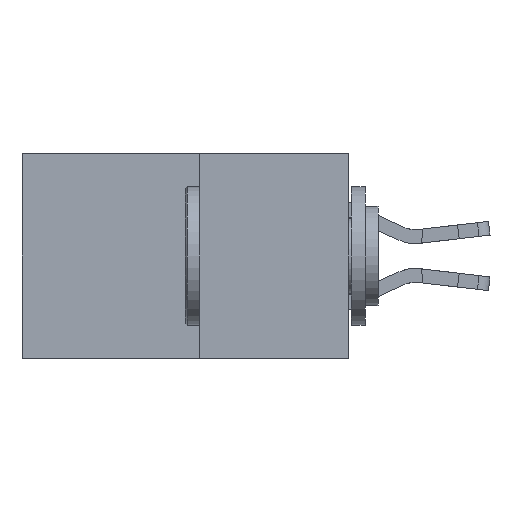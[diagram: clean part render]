
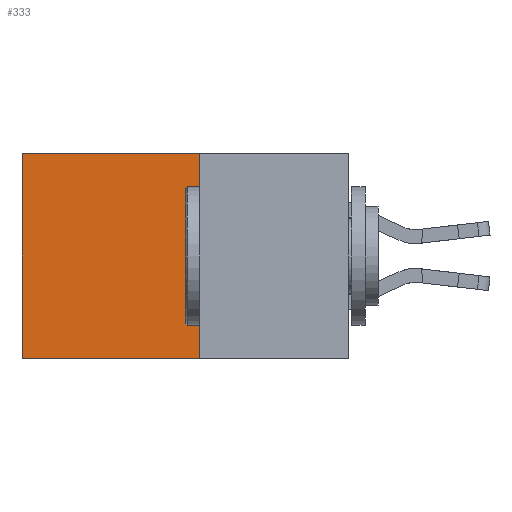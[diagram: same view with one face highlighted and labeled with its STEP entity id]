
A CAD part, left-side view. The second image highlights one B-rep face of the part: STEP entity #333.
In plain terms, the highlighted planar face has unit normal (-1, 0, 0).
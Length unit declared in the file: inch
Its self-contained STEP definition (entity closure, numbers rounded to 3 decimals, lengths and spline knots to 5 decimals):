
#333 = ADVANCED_FACE ( 'NONE', ( #1556 ), #15491, .F. ) ;
#645 = CARTESIAN_POINT ( 'NONE',  ( 0.277, 0.27, 0. ) ) ;
#831 = DIRECTION ( 'NONE',  ( 0., 0., -1. ) ) ;
#1556 = FACE_OUTER_BOUND ( 'NONE', #3323, .T. ) ;
#1983 = LINE ( 'NONE', #10233, #12766 ) ;
#2122 = EDGE_CURVE ( 'NONE', #16113, #11351, #10534, .T. ) ;
#2953 = CARTESIAN_POINT ( 'NONE',  ( 0.277, 0.59, -0.37 ) ) ;
#3068 = CARTESIAN_POINT ( 'NONE',  ( 0.277, 0.27, 0. ) ) ;
#3210 = VECTOR ( 'NONE', #16362, 39.37008 ) ;
#3323 = EDGE_LOOP ( 'NONE', ( #10973, #4220, #12655, #10870 ) ) ;
#3416 = CARTESIAN_POINT ( 'NONE',  ( 0.277, 0.27, -0.37 ) ) ;
#4220 = ORIENTED_EDGE ( 'NONE', *, *, #7150, .F. ) ;
#4374 = DIRECTION ( 'NONE',  ( 0., 1., 0. ) ) ;
#6694 = CARTESIAN_POINT ( 'NONE',  ( 0.277, 0.59, 0. ) ) ;
#7150 = EDGE_CURVE ( 'NONE', #10003, #11351, #1983, .T. ) ;
#7243 = DIRECTION ( 'NONE',  ( 1., 0., 0. ) ) ;
#7878 = VECTOR ( 'NONE', #11225, 39.37008 ) ;
#8454 = EDGE_CURVE ( 'NONE', #13635, #10003, #13472, .T. ) ;
#10003 = VERTEX_POINT ( 'NONE', #13019 ) ;
#10208 = DIRECTION ( 'NONE',  ( 0., 1., 0. ) ) ;
#10232 = EDGE_CURVE ( 'NONE', #13635, #16113, #10466, .T. ) ;
#10233 = CARTESIAN_POINT ( 'NONE',  ( 0.277, 0.27, -0.37 ) ) ;
#10466 = LINE ( 'NONE', #3068, #16575 ) ;
#10534 = LINE ( 'NONE', #2953, #3210 ) ;
#10870 = ORIENTED_EDGE ( 'NONE', *, *, #10232, .T. ) ;
#10973 = ORIENTED_EDGE ( 'NONE', *, *, #2122, .T. ) ;
#11037 = AXIS2_PLACEMENT_3D ( 'NONE', #11096, #7243, #831 ) ;
#11096 = CARTESIAN_POINT ( 'NONE',  ( 0.277, 0.27, -0.37 ) ) ;
#11225 = DIRECTION ( 'NONE',  ( 0., 0., -1. ) ) ;
#11351 = VERTEX_POINT ( 'NONE', #14270 ) ;
#12655 = ORIENTED_EDGE ( 'NONE', *, *, #8454, .F. ) ;
#12766 = VECTOR ( 'NONE', #10208, 39.37008 ) ;
#13019 = CARTESIAN_POINT ( 'NONE',  ( 0.277, 0.27, -0.37 ) ) ;
#13472 = LINE ( 'NONE', #3416, #7878 ) ;
#13635 = VERTEX_POINT ( 'NONE', #645 ) ;
#14270 = CARTESIAN_POINT ( 'NONE',  ( 0.277, 0.59, -0.37 ) ) ;
#15491 = PLANE ( 'NONE',  #11037 ) ;
#16113 = VERTEX_POINT ( 'NONE', #6694 ) ;
#16362 = DIRECTION ( 'NONE',  ( 0., 0., -1. ) ) ;
#16575 = VECTOR ( 'NONE', #4374, 39.37008 ) ;
